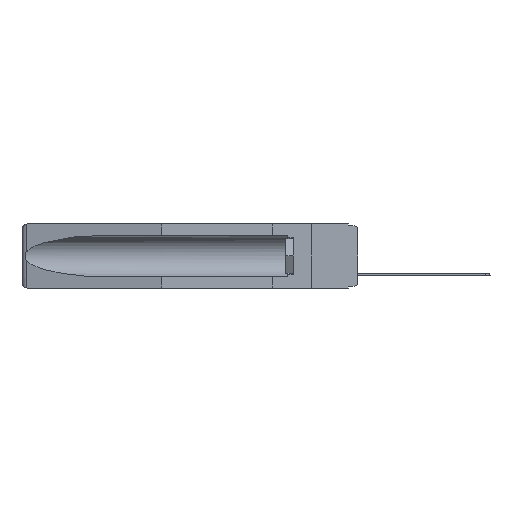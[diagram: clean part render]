
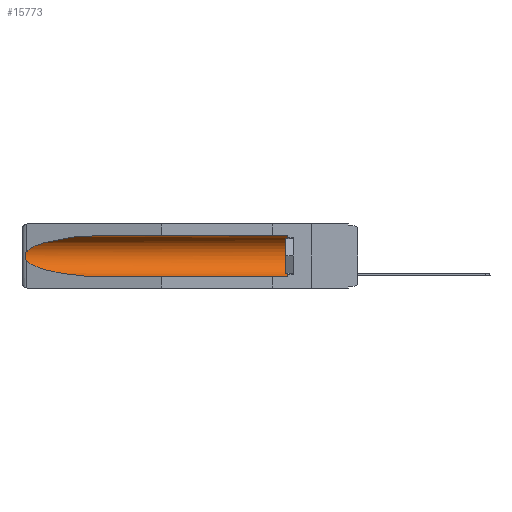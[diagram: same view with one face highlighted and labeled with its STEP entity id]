
A CAD part, left-side view. The second image highlights one B-rep face of the part: STEP entity #15773.
In plain terms, the highlighted cylindrical face has radius 2.857 mm (diameter 5.715 mm), a partial arc.
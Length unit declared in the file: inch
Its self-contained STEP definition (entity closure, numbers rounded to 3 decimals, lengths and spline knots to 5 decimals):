
#278 = FACE_OUTER_BOUND ( 'NONE', #6996, .T. ) ;
#298 = DIRECTION ( 'NONE',  ( 0., 1., 0. ) ) ;
#465 =( BOUNDED_CURVE ( )  B_SPLINE_CURVE ( 3, ( #5285, #535, #6772, #5162 ),
 .UNSPECIFIED., .F., .F. ) 
 B_SPLINE_CURVE_WITH_KNOTS ( ( 4, 4 ),
 ( 0.1948, 1.5708 ),
 .UNSPECIFIED. ) 
 CURVE ( )  GEOMETRIC_REPRESENTATION_ITEM ( )  RATIONAL_B_SPLINE_CURVE ( ( 1., 0.848, 0.848, 1. ) ) 
 REPRESENTATION_ITEM ( '' )  );
#535 = CARTESIAN_POINT ( 'NONE',  ( 0.25451, 1.48313, -0.24835 ) ) ;
#792 = ORIENTED_EDGE ( 'NONE', *, *, #14368, .T. ) ;
#1180 = CARTESIAN_POINT ( 'NONE',  ( 0.25451, 1.48313, -0.09465 ) ) ;
#1258 = CARTESIAN_POINT ( 'NONE',  ( 0.2673, 1.5327, -0.16383 ) ) ;
#2061 = AXIS2_PLACEMENT_3D ( 'NONE', #15822, #15689, #8361 ) ;
#2402 = LINE ( 'NONE', #5835, #9841 ) ;
#2532 = VERTEX_POINT ( 'NONE', #11634 ) ;
#2780 = CARTESIAN_POINT ( 'NONE',  ( 0.2673, 1.53269, -0.17917 ) ) ;
#3310 = CARTESIAN_POINT ( 'NONE',  ( 0.155, -0.30754, -0.1715 ) ) ;
#3363 = AXIS2_PLACEMENT_3D ( 'NONE', #3310, #298, #18250 ) ;
#3948 =( BOUNDED_CURVE ( )  B_SPLINE_CURVE ( 3, ( #11528, #4131, #1180, #6837 ),
 .UNSPECIFIED., .F., .F. ) 
 B_SPLINE_CURVE_WITH_KNOTS ( ( 4, 4 ),
 ( 4.71239, 6.08839 ),
 .UNSPECIFIED. ) 
 CURVE ( )  GEOMETRIC_REPRESENTATION_ITEM ( )  RATIONAL_B_SPLINE_CURVE ( ( 1., 0.848, 0.848, 1. ) ) 
 REPRESENTATION_ITEM ( '' )  );
#3949 = ORIENTED_EDGE ( 'NONE', *, *, #10918, .T. ) ;
#4131 = CARTESIAN_POINT ( 'NONE',  ( 0.21114, 1.30732, -0.059 ) ) ;
#4260 = CARTESIAN_POINT ( 'NONE',  ( 0.26655, 1.53094, -0.18657 ) ) ;
#4897 = EDGE_CURVE ( 'NONE', #10043, #15478, #3948, .T. ) ;
#5162 = CARTESIAN_POINT ( 'NONE',  ( 0.155, 1.07973, -0.284 ) ) ;
#5285 = CARTESIAN_POINT ( 'NONE',  ( 0.26537, 1.52718, -0.19328 ) ) ;
#5835 = CARTESIAN_POINT ( 'NONE',  ( 0.155, -0.30754, -0.284 ) ) ;
#6772 = CARTESIAN_POINT ( 'NONE',  ( 0.21114, 1.30732, -0.284 ) ) ;
#6837 = CARTESIAN_POINT ( 'NONE',  ( 0.26537, 1.52718, -0.14972 ) ) ;
#6996 = EDGE_LOOP ( 'NONE', ( #12945, #792, #17070, #15297, #3949, #8843 ) ) ;
#7174 = CARTESIAN_POINT ( 'NONE',  ( 0.26537, 1.52718, -0.14972 ) ) ;
#7987 = EDGE_CURVE ( 'NONE', #17639, #10043, #14810, .T. ) ;
#8361 = DIRECTION ( 'NONE',  ( 0., 0., 1. ) ) ;
#8767 = CARTESIAN_POINT ( 'NONE',  ( 0.26537, 1.52718, -0.14972 ) ) ;
#8843 = ORIENTED_EDGE ( 'NONE', *, *, #7987, .T. ) ;
#8894 = DIRECTION ( 'NONE',  ( 0., 1., 0. ) ) ;
#9841 = VECTOR ( 'NONE', #8894, 39.37008 ) ;
#9982 = CARTESIAN_POINT ( 'NONE',  ( 0.155, 0.126, -0.284 ) ) ;
#10043 = VERTEX_POINT ( 'NONE', #10522 ) ;
#10181 = CARTESIAN_POINT ( 'NONE',  ( 0.26654, 1.53092, -0.15636 ) ) ;
#10522 = CARTESIAN_POINT ( 'NONE',  ( 0.155, 1.07973, -0.059 ) ) ;
#10918 = EDGE_CURVE ( 'NONE', #12893, #17639, #11043, .T. ) ;
#11043 = CIRCLE ( 'NONE', #2061, 0.1125 ) ;
#11378 = CARTESIAN_POINT ( 'NONE',  ( 0.155, -0.30754, -0.059 ) ) ;
#11412 = EDGE_CURVE ( 'NONE', #12893, #17628, #2402, .T. ) ;
#11528 = CARTESIAN_POINT ( 'NONE',  ( 0.155, 1.07973, -0.059 ) ) ;
#11634 = CARTESIAN_POINT ( 'NONE',  ( 0.26537, 1.52718, -0.19328 ) ) ;
#11671 = CARTESIAN_POINT ( 'NONE',  ( 0.2675, 1.53308, -0.16763 ) ) ;
#12824 = DIRECTION ( 'NONE',  ( 0., 1., 0. ) ) ;
#12893 = VERTEX_POINT ( 'NONE', #9982 ) ;
#12945 = ORIENTED_EDGE ( 'NONE', *, *, #4897, .T. ) ;
#14368 = EDGE_CURVE ( 'NONE', #15478, #2532, #17221, .T. ) ;
#14695 = CARTESIAN_POINT ( 'NONE',  ( 0.26537, 1.52718, -0.19328 ) ) ;
#14810 = LINE ( 'NONE', #11378, #17386 ) ;
#14876 = CARTESIAN_POINT ( 'NONE',  ( 0.26597, 1.52961, -0.15275 ) ) ;
#15297 = ORIENTED_EDGE ( 'NONE', *, *, #11412, .F. ) ;
#15478 = VERTEX_POINT ( 'NONE', #8767 ) ;
#15689 = DIRECTION ( 'NONE',  ( 0., -1., 0. ) ) ;
#15773 = ADVANCED_FACE ( 'NONE', ( #278 ), #19190, .F. ) ;
#15822 = CARTESIAN_POINT ( 'NONE',  ( 0.155, 0.126, -0.1715 ) ) ;
#17070 = ORIENTED_EDGE ( 'NONE', *, *, #18820, .T. ) ;
#17160 = CARTESIAN_POINT ( 'NONE',  ( 0.155, 0.126, -0.059 ) ) ;
#17221 = B_SPLINE_CURVE_WITH_KNOTS ( 'NONE', 3,
 ( #7174, #14876, #10181, #1258, #11671, #17699, #2780, #4260, #19195, #14695 ),
 .UNSPECIFIED., .F., .F.,
 ( 4, 2, 2, 2, 4 ),
 ( 0., 0.00029, 0.00058, 0.00087, 0.00117 ),
 .UNSPECIFIED. ) ;
#17386 = VECTOR ( 'NONE', #12824, 39.37008 ) ;
#17628 = VERTEX_POINT ( 'NONE', #18852 ) ;
#17639 = VERTEX_POINT ( 'NONE', #17160 ) ;
#17699 = CARTESIAN_POINT ( 'NONE',  ( 0.2675, 1.53308, -0.17534 ) ) ;
#18250 = DIRECTION ( 'NONE',  ( 0., 0., 1. ) ) ;
#18820 = EDGE_CURVE ( 'NONE', #2532, #17628, #465, .T. ) ;
#18852 = CARTESIAN_POINT ( 'NONE',  ( 0.155, 1.07973, -0.284 ) ) ;
#19190 = CYLINDRICAL_SURFACE ( 'NONE', #3363, 0.1125 ) ;
#19195 = CARTESIAN_POINT ( 'NONE',  ( 0.26597, 1.5296, -0.19026 ) ) ;
